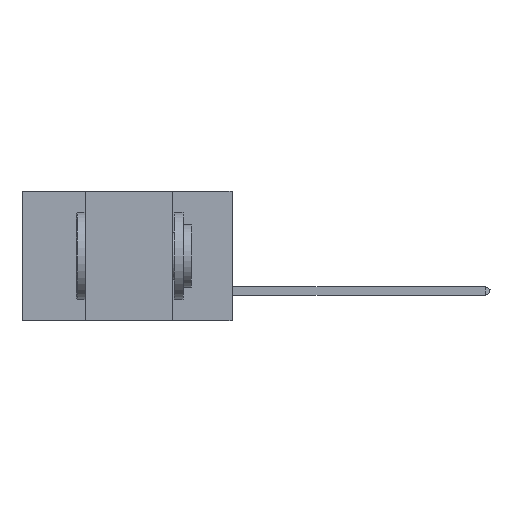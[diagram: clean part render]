
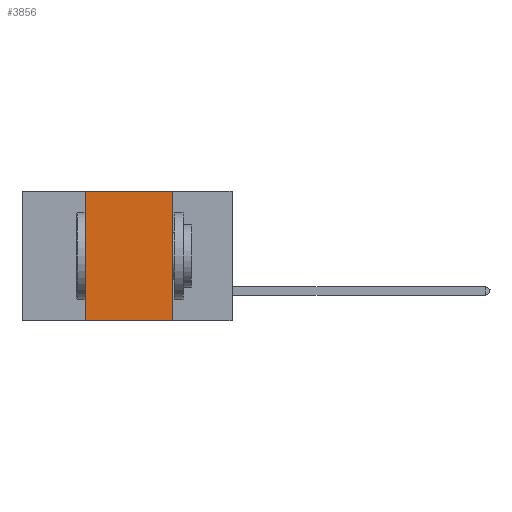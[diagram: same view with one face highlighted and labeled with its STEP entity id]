
A CAD part, left-side view. The second image highlights one B-rep face of the part: STEP entity #3856.
In plain terms, the highlighted planar face has unit normal (-1, 0, 0).
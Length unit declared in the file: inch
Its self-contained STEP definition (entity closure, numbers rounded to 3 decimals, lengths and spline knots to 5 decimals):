
#2786 = EDGE_CURVE ( 'NONE', #17300, #15036, #26878, .T. ) ;
#3232 = ORIENTED_EDGE ( 'NONE', *, *, #7158, .F. ) ;
#3856 = ADVANCED_FACE ( 'NONE', ( #6796 ), #22579, .F. ) ;
#4116 = DIRECTION ( 'NONE',  ( 0., -1., 0. ) ) ;
#5928 = VECTOR ( 'NONE', #28247, 39.37008 ) ;
#6267 = CARTESIAN_POINT ( 'NONE',  ( 0., 0.42, 0. ) ) ;
#6796 = FACE_OUTER_BOUND ( 'NONE', #20320, .T. ) ;
#7158 = EDGE_CURVE ( 'NONE', #35863, #15279, #7618, .T. ) ;
#7618 = LINE ( 'NONE', #27800, #34651 ) ;
#13676 = CARTESIAN_POINT ( 'NONE',  ( 0., 0.17, -0.37 ) ) ;
#14169 = CARTESIAN_POINT ( 'NONE',  ( 0., 0.6, 0. ) ) ;
#15036 = VERTEX_POINT ( 'NONE', #6267 ) ;
#15279 = VERTEX_POINT ( 'NONE', #13676 ) ;
#17300 = VERTEX_POINT ( 'NONE', #23709 ) ;
#19029 = VECTOR ( 'NONE', #33527, 39.37008 ) ;
#19223 = ORIENTED_EDGE ( 'NONE', *, *, #28236, .T. ) ;
#20320 = EDGE_LOOP ( 'NONE', ( #3232, #28553, #30325, #19223 ) ) ;
#21975 = DIRECTION ( 'NONE',  ( 0., 0., -1. ) ) ;
#22579 = PLANE ( 'NONE',  #24623 ) ;
#22886 = LINE ( 'NONE', #25592, #5928 ) ;
#23215 = EDGE_CURVE ( 'NONE', #15036, #35863, #22886, .T. ) ;
#23709 = CARTESIAN_POINT ( 'NONE',  ( 0., 0.42, -0.37 ) ) ;
#23788 = CARTESIAN_POINT ( 'NONE',  ( 0., 0.17, 0. ) ) ;
#24623 = AXIS2_PLACEMENT_3D ( 'NONE', #14169, #28294, #34097 ) ;
#25592 = CARTESIAN_POINT ( 'NONE',  ( 0., 0.6, 0. ) ) ;
#26878 = LINE ( 'NONE', #31109, #19029 ) ;
#27800 = CARTESIAN_POINT ( 'NONE',  ( 0., 0.17, 0. ) ) ;
#28236 = EDGE_CURVE ( 'NONE', #17300, #15279, #29087, .T. ) ;
#28247 = DIRECTION ( 'NONE',  ( 0., -1., 0. ) ) ;
#28294 = DIRECTION ( 'NONE',  ( 1., 0., 0. ) ) ;
#28553 = ORIENTED_EDGE ( 'NONE', *, *, #23215, .F. ) ;
#29087 = LINE ( 'NONE', #29278, #35712 ) ;
#29278 = CARTESIAN_POINT ( 'NONE',  ( 0., 0.6, -0.37 ) ) ;
#30325 = ORIENTED_EDGE ( 'NONE', *, *, #2786, .F. ) ;
#31109 = CARTESIAN_POINT ( 'NONE',  ( 0., 0.42, 0. ) ) ;
#33527 = DIRECTION ( 'NONE',  ( 0., 0., 1. ) ) ;
#34097 = DIRECTION ( 'NONE',  ( 0., 0., -1. ) ) ;
#34651 = VECTOR ( 'NONE', #21975, 39.37008 ) ;
#35712 = VECTOR ( 'NONE', #4116, 39.37008 ) ;
#35863 = VERTEX_POINT ( 'NONE', #23788 ) ;
